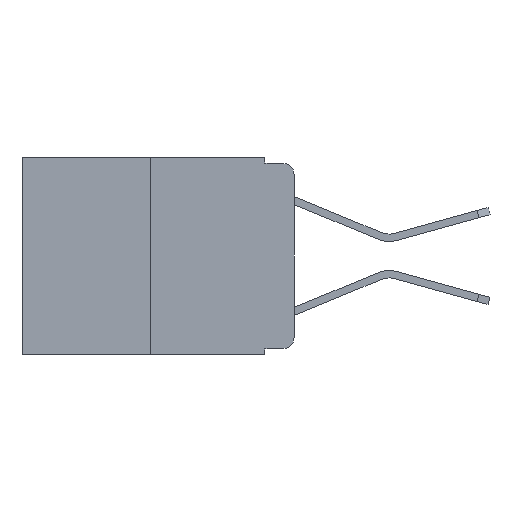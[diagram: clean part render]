
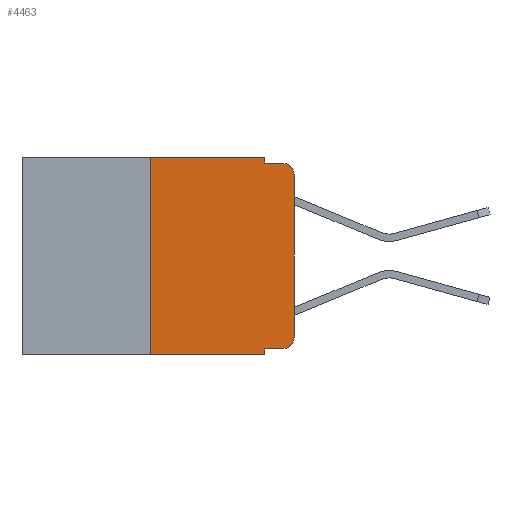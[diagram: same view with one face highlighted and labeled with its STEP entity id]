
A CAD part, left-side view. The second image highlights one B-rep face of the part: STEP entity #4463.
In plain terms, the highlighted planar face has unit normal (-1, 0, 0).
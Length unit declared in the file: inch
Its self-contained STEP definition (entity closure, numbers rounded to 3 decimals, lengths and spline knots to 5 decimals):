
#295 = VERTEX_POINT ( 'NONE', #7869 ) ;
#410 = LINE ( 'NONE', #11488, #4815 ) ;
#943 = CARTESIAN_POINT ( 'NONE',  ( 0., 0., 0. ) ) ;
#1240 = CARTESIAN_POINT ( 'NONE',  ( 0., 0.02, -0.313 ) ) ;
#1299 = VECTOR ( 'NONE', #10134, 39.37008 ) ;
#2003 = CARTESIAN_POINT ( 'NONE',  ( 0., 0.25, -0.343 ) ) ;
#2625 = DIRECTION ( 'NONE',  ( 0., 0., -1. ) ) ;
#2873 = ORIENTED_EDGE ( 'NONE', *, *, #11491, .T. ) ;
#3298 = ORIENTED_EDGE ( 'NONE', *, *, #9664, .F. ) ;
#3370 = PLANE ( 'NONE',  #4812 ) ;
#3804 = CARTESIAN_POINT ( 'NONE',  ( 0., 0.02, -0.03 ) ) ;
#3905 = DIRECTION ( 'NONE',  ( 0., 0., -1. ) ) ;
#4011 = DIRECTION ( 'NONE',  ( 0., -1., 0. ) ) ;
#4037 = LINE ( 'NONE', #12736, #7352 ) ;
#4111 = ORIENTED_EDGE ( 'NONE', *, *, #11559, .T. ) ;
#4150 = VERTEX_POINT ( 'NONE', #12973 ) ;
#4177 = CARTESIAN_POINT ( 'NONE',  ( 0., 0., -0.03 ) ) ;
#4285 = DIRECTION ( 'NONE',  ( 0., 0., -1. ) ) ;
#4415 = LINE ( 'NONE', #6392, #11152 ) ;
#4463 = ADVANCED_FACE ( 'NONE', ( #12884 ), #3370, .F. ) ;
#4506 = ORIENTED_EDGE ( 'NONE', *, *, #11580, .T. ) ;
#4812 = AXIS2_PLACEMENT_3D ( 'NONE', #11286, #12658, #4285 ) ;
#4815 = VECTOR ( 'NONE', #3905, 39.37008 ) ;
#4911 = VERTEX_POINT ( 'NONE', #11609 ) ;
#5063 = DIRECTION ( 'NONE',  ( 0., 0., -1. ) ) ;
#5265 = CARTESIAN_POINT ( 'NONE',  ( 0., 0.473, 0. ) ) ;
#5497 = VERTEX_POINT ( 'NONE', #4177 ) ;
#6392 = CARTESIAN_POINT ( 'NONE',  ( 0., 0.25, 0. ) ) ;
#7352 = VECTOR ( 'NONE', #13950, 39.37008 ) ;
#7557 = DIRECTION ( 'NONE',  ( 0., -1., 0. ) ) ;
#7743 = VECTOR ( 'NONE', #7557, 39.37008 ) ;
#7860 = VECTOR ( 'NONE', #13725, 39.37008 ) ;
#7869 = CARTESIAN_POINT ( 'NONE',  ( 0., 0.051, -0.333 ) ) ;
#7935 = VERTEX_POINT ( 'NONE', #2003 ) ;
#8135 = LINE ( 'NONE', #13850, #7743 ) ;
#8233 = EDGE_LOOP ( 'NONE', ( #2873, #9600, #12988, #16093, #3298, #10018, #10428, #13750, #4111, #4506 ) ) ;
#8243 = LINE ( 'NONE', #12500, #7860 ) ;
#8656 = DIRECTION ( 'NONE',  ( 0., 0., 1. ) ) ;
#9055 = CARTESIAN_POINT ( 'NONE',  ( 0., 0.051, -0.343 ) ) ;
#9600 = ORIENTED_EDGE ( 'NONE', *, *, #11516, .T. ) ;
#9659 = VECTOR ( 'NONE', #4011, 39.37008 ) ;
#9664 = EDGE_CURVE ( 'NONE', #13944, #11977, #16143, .T. ) ;
#9731 = CARTESIAN_POINT ( 'NONE',  ( 0., 0.02, -0.333 ) ) ;
#9922 = EDGE_CURVE ( 'NONE', #7935, #11620, #8243, .T. ) ;
#9941 = CARTESIAN_POINT ( 'NONE',  ( 0., 0.051, 0. ) ) ;
#10018 = ORIENTED_EDGE ( 'NONE', *, *, #11539, .F. ) ;
#10065 = VERTEX_POINT ( 'NONE', #14029 ) ;
#10088 = AXIS2_PLACEMENT_3D ( 'NONE', #3804, #12627, #5063 ) ;
#10134 = DIRECTION ( 'NONE',  ( 0., 0., -1. ) ) ;
#10240 = DIRECTION ( 'NONE',  ( -1., 0., 0. ) ) ;
#10428 = ORIENTED_EDGE ( 'NONE', *, *, #9922, .T. ) ;
#10938 = AXIS2_PLACEMENT_3D ( 'NONE', #1240, #10240, #2625 ) ;
#11152 = VECTOR ( 'NONE', #15105, 39.37008 ) ;
#11286 = CARTESIAN_POINT ( 'NONE',  ( 0., 0.473, 0. ) ) ;
#11488 = CARTESIAN_POINT ( 'NONE',  ( 0., 0.051, 0. ) ) ;
#11491 = EDGE_CURVE ( 'NONE', #10065, #5497, #12336, .T. ) ;
#11516 = EDGE_CURVE ( 'NONE', #5497, #4150, #11938, .T. ) ;
#11532 = EDGE_CURVE ( 'NONE', #4911, #4150, #8135, .T. ) ;
#11536 = EDGE_CURVE ( 'NONE', #11977, #4911, #14417, .T. ) ;
#11539 = EDGE_CURVE ( 'NONE', #7935, #13944, #4415, .T. ) ;
#11555 = EDGE_CURVE ( 'NONE', #295, #11620, #410, .T. ) ;
#11559 = EDGE_CURVE ( 'NONE', #295, #14118, #4037, .T. ) ;
#11580 = EDGE_CURVE ( 'NONE', #14118, #10065, #13672, .T. ) ;
#11609 = CARTESIAN_POINT ( 'NONE',  ( 0., 0.051, -0.01 ) ) ;
#11620 = VERTEX_POINT ( 'NONE', #9055 ) ;
#11938 = CIRCLE ( 'NONE', #10088, 0.02 ) ;
#11977 = VERTEX_POINT ( 'NONE', #9941 ) ;
#12336 = LINE ( 'NONE', #943, #15179 ) ;
#12500 = CARTESIAN_POINT ( 'NONE',  ( 0., 0.473, -0.343 ) ) ;
#12627 = DIRECTION ( 'NONE',  ( -1., 0., 0. ) ) ;
#12658 = DIRECTION ( 'NONE',  ( 1., 0., 0. ) ) ;
#12736 = CARTESIAN_POINT ( 'NONE',  ( 0., 0.051, -0.333 ) ) ;
#12884 = FACE_OUTER_BOUND ( 'NONE', #8233, .T. ) ;
#12973 = CARTESIAN_POINT ( 'NONE',  ( 0., 0.02, -0.01 ) ) ;
#12988 = ORIENTED_EDGE ( 'NONE', *, *, #11532, .F. ) ;
#13672 = CIRCLE ( 'NONE', #10938, 0.02 ) ;
#13725 = DIRECTION ( 'NONE',  ( 0., -1., 0. ) ) ;
#13750 = ORIENTED_EDGE ( 'NONE', *, *, #11555, .F. ) ;
#13850 = CARTESIAN_POINT ( 'NONE',  ( 0., 0.051, -0.01 ) ) ;
#13944 = VERTEX_POINT ( 'NONE', #15434 ) ;
#13950 = DIRECTION ( 'NONE',  ( 0., -1., 0. ) ) ;
#14029 = CARTESIAN_POINT ( 'NONE',  ( 0., 0., -0.313 ) ) ;
#14118 = VERTEX_POINT ( 'NONE', #9731 ) ;
#14417 = LINE ( 'NONE', #16166, #1299 ) ;
#15105 = DIRECTION ( 'NONE',  ( 0., 0., 1. ) ) ;
#15179 = VECTOR ( 'NONE', #8656, 39.37008 ) ;
#15434 = CARTESIAN_POINT ( 'NONE',  ( 0., 0.25, 0. ) ) ;
#16093 = ORIENTED_EDGE ( 'NONE', *, *, #11536, .F. ) ;
#16143 = LINE ( 'NONE', #5265, #9659 ) ;
#16166 = CARTESIAN_POINT ( 'NONE',  ( 0., 0.051, 0. ) ) ;
